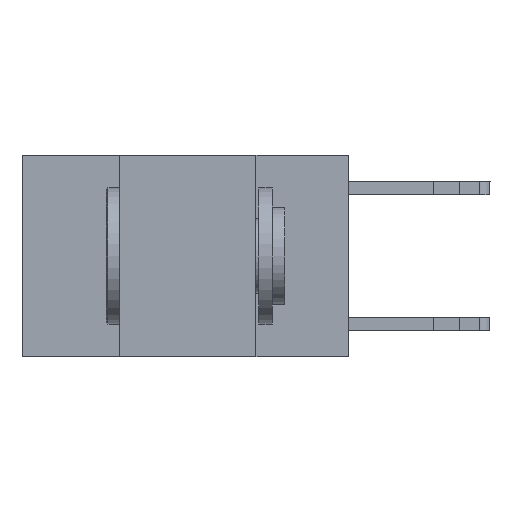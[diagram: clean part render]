
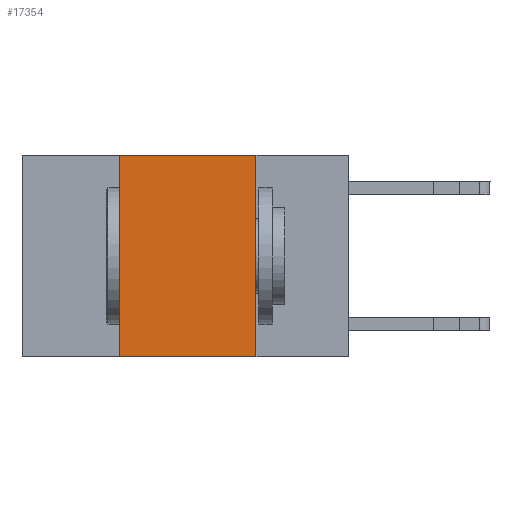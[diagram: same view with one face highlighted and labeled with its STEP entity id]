
A CAD part, left-side view. The second image highlights one B-rep face of the part: STEP entity #17354.
In plain terms, the highlighted planar face has unit normal (-1, 0, 0).
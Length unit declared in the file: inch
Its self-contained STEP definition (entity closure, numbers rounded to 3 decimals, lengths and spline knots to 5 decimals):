
#70 = EDGE_LOOP ( 'NONE', ( #7106, #4570, #12206, #3896 ) ) ;
#558 = AXIS2_PLACEMENT_3D ( 'NONE', #17892, #5793, #1524 ) ;
#584 = DIRECTION ( 'NONE',  ( 0., -1., 0. ) ) ;
#783 = CARTESIAN_POINT ( 'NONE',  ( 0., 0.17, 0. ) ) ;
#1524 = DIRECTION ( 'NONE',  ( 0., 0., -1. ) ) ;
#2044 = DIRECTION ( 'NONE',  ( 0., 0., -1. ) ) ;
#2385 = CARTESIAN_POINT ( 'NONE',  ( 0., 0.42, 0. ) ) ;
#2587 = CARTESIAN_POINT ( 'NONE',  ( 0., 0.6, -0.37 ) ) ;
#3896 = ORIENTED_EDGE ( 'NONE', *, *, #14114, .T. ) ;
#4570 = ORIENTED_EDGE ( 'NONE', *, *, #6350, .F. ) ;
#4902 = EDGE_CURVE ( 'NONE', #6568, #14832, #8128, .T. ) ;
#5793 = DIRECTION ( 'NONE',  ( 1., 0., 0. ) ) ;
#6350 = EDGE_CURVE ( 'NONE', #14832, #18720, #17026, .T. ) ;
#6568 = VERTEX_POINT ( 'NONE', #7180 ) ;
#6682 = CARTESIAN_POINT ( 'NONE',  ( 0., 0.6, 0. ) ) ;
#7106 = ORIENTED_EDGE ( 'NONE', *, *, #15289, .F. ) ;
#7180 = CARTESIAN_POINT ( 'NONE',  ( 0., 0.42, -0.37 ) ) ;
#8128 = LINE ( 'NONE', #2385, #9211 ) ;
#8838 = VERTEX_POINT ( 'NONE', #16370 ) ;
#9211 = VECTOR ( 'NONE', #11137, 39.37008 ) ;
#10207 = VECTOR ( 'NONE', #16314, 39.37008 ) ;
#10352 = LINE ( 'NONE', #2587, #10207 ) ;
#11080 = VECTOR ( 'NONE', #584, 39.37008 ) ;
#11137 = DIRECTION ( 'NONE',  ( 0., 0., 1. ) ) ;
#11566 = CARTESIAN_POINT ( 'NONE',  ( 0., 0.17, 0. ) ) ;
#12206 = ORIENTED_EDGE ( 'NONE', *, *, #4902, .F. ) ;
#12732 = VECTOR ( 'NONE', #2044, 39.37008 ) ;
#13809 = LINE ( 'NONE', #783, #12732 ) ;
#14114 = EDGE_CURVE ( 'NONE', #6568, #8838, #10352, .T. ) ;
#14832 = VERTEX_POINT ( 'NONE', #18543 ) ;
#14838 = FACE_OUTER_BOUND ( 'NONE', #70, .T. ) ;
#14947 = PLANE ( 'NONE',  #558 ) ;
#15289 = EDGE_CURVE ( 'NONE', #18720, #8838, #13809, .T. ) ;
#16314 = DIRECTION ( 'NONE',  ( 0., -1., 0. ) ) ;
#16370 = CARTESIAN_POINT ( 'NONE',  ( 0., 0.17, -0.37 ) ) ;
#17026 = LINE ( 'NONE', #6682, #11080 ) ;
#17354 = ADVANCED_FACE ( 'NONE', ( #14838 ), #14947, .F. ) ;
#17892 = CARTESIAN_POINT ( 'NONE',  ( 0., 0.6, 0. ) ) ;
#18543 = CARTESIAN_POINT ( 'NONE',  ( 0., 0.42, 0. ) ) ;
#18720 = VERTEX_POINT ( 'NONE', #11566 ) ;
